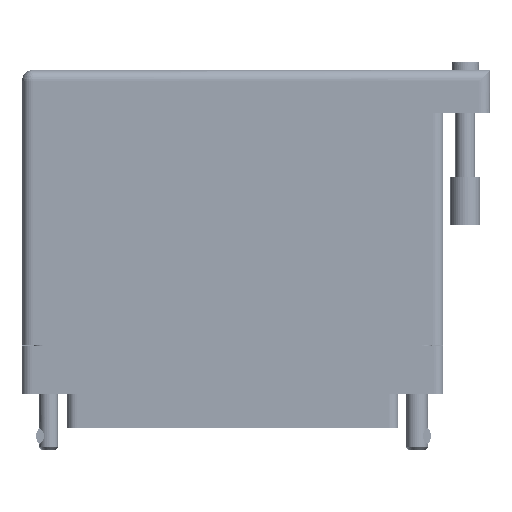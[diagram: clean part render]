
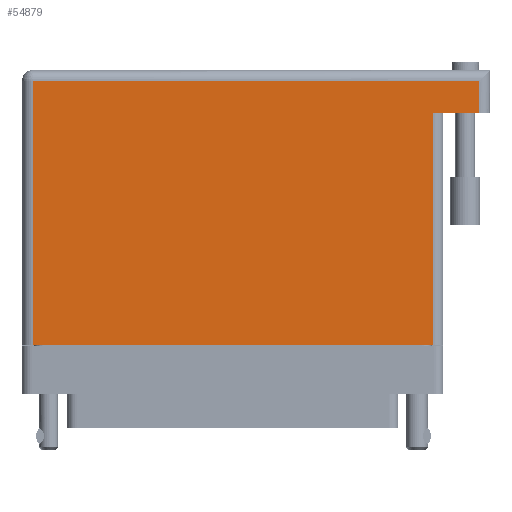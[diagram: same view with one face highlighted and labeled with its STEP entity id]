
A CAD part, front view. The second image highlights one B-rep face of the part: STEP entity #54879.
In plain terms, the highlighted face is planar.
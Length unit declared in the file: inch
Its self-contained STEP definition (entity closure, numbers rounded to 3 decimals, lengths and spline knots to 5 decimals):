
#2619 = DIRECTION ( 'NONE',  ( 0., 0., -1. ) ) ;
#3626 = CARTESIAN_POINT ( 'NONE',  ( 1.589, 1.605, 0.617 ) ) ;
#3721 = DIRECTION ( 'NONE',  ( 1., 0., 0. ) ) ;
#5409 = DIRECTION ( 'NONE',  ( -1., 0., 0. ) ) ;
#10530 = VECTOR ( 'NONE', #23652, 39.37008 ) ;
#10842 = LINE ( 'NONE', #23153, #66953 ) ;
#14920 = DIRECTION ( 'NONE',  ( -1., 0., 0. ) ) ;
#15500 = CARTESIAN_POINT ( 'NONE',  ( 1.289, -0.1, 0.617 ) ) ;
#17775 = CARTESIAN_POINT ( 'NONE',  ( 1.289, 1.395, 0.617 ) ) ;
#20350 = VERTEX_POINT ( 'NONE', #54851 ) ;
#20756 = EDGE_CURVE ( 'NONE', #31509, #25315, #49983, .T. ) ;
#21110 = LINE ( 'NONE', #66431, #63501 ) ;
#22135 = PLANE ( 'NONE',  #81626 ) ;
#23153 = CARTESIAN_POINT ( 'NONE',  ( 1.659, 1.395, 0.617 ) ) ;
#23652 = DIRECTION ( 'NONE',  ( 0., -1., 0. ) ) ;
#24788 = VERTEX_POINT ( 'NONE', #55376 ) ;
#25315 = VERTEX_POINT ( 'NONE', #38615 ) ;
#27882 = DIRECTION ( 'NONE',  ( 0., 1., 0. ) ) ;
#28761 = CARTESIAN_POINT ( 'NONE',  ( -1.289, 1.605, 0.617 ) ) ;
#31509 = VERTEX_POINT ( 'NONE', #15500 ) ;
#38293 = EDGE_LOOP ( 'NONE', ( #81218, #76548, #80251, #51467, #76571, #50069 ) ) ;
#38615 = CARTESIAN_POINT ( 'NONE',  ( 1.289, 1.395, 0.617 ) ) ;
#39125 = EDGE_CURVE ( 'NONE', #20350, #25315, #10842, .T. ) ;
#41628 = EDGE_CURVE ( 'NONE', #69132, #62494, #77031, .T. ) ;
#42671 = VECTOR ( 'NONE', #69472, 39.37008 ) ;
#49983 = LINE ( 'NONE', #17775, #42671 ) ;
#50069 = ORIENTED_EDGE ( 'NONE', *, *, #62685, .T. ) ;
#50326 = LINE ( 'NONE', #55845, #10530 ) ;
#50994 = VECTOR ( 'NONE', #5409, 39.37008 ) ;
#51467 = ORIENTED_EDGE ( 'NONE', *, *, #78425, .T. ) ;
#54851 = CARTESIAN_POINT ( 'NONE',  ( 1.589, 1.395, 0.617 ) ) ;
#54879 = ADVANCED_FACE ( 'NONE', ( #55159 ), #22135, .F. ) ;
#55159 = FACE_OUTER_BOUND ( 'NONE', #38293, .T. ) ;
#55376 = CARTESIAN_POINT ( 'NONE',  ( -1.289, -0.1, 0.617 ) ) ;
#55845 = CARTESIAN_POINT ( 'NONE',  ( -1.289, -0.1, 0.617 ) ) ;
#62494 = VERTEX_POINT ( 'NONE', #28761 ) ;
#62611 = EDGE_CURVE ( 'NONE', #24788, #31509, #74917, .T. ) ;
#62685 = EDGE_CURVE ( 'NONE', #62494, #24788, #50326, .T. ) ;
#63501 = VECTOR ( 'NONE', #27882, 39.37008 ) ;
#66431 = CARTESIAN_POINT ( 'NONE',  ( 1.589, 1.675, 0.617 ) ) ;
#66953 = VECTOR ( 'NONE', #68909, 39.37008 ) ;
#68909 = DIRECTION ( 'NONE',  ( -1., 0., 0. ) ) ;
#69132 = VERTEX_POINT ( 'NONE', #3626 ) ;
#69472 = DIRECTION ( 'NONE',  ( 0., 1., 0. ) ) ;
#72820 = VECTOR ( 'NONE', #3721, 39.37008 ) ;
#74917 = LINE ( 'NONE', #81711, #72820 ) ;
#76548 = ORIENTED_EDGE ( 'NONE', *, *, #20756, .T. ) ;
#76571 = ORIENTED_EDGE ( 'NONE', *, *, #41628, .T. ) ;
#76600 = CARTESIAN_POINT ( 'NONE',  ( -1.359, 1.605, 0.617 ) ) ;
#77031 = LINE ( 'NONE', #76600, #50994 ) ;
#78425 = EDGE_CURVE ( 'NONE', #20350, #69132, #21110, .T. ) ;
#80251 = ORIENTED_EDGE ( 'NONE', *, *, #39125, .F. ) ;
#81033 = CARTESIAN_POINT ( 'NONE',  ( -1.359, 1.675, 0.617 ) ) ;
#81218 = ORIENTED_EDGE ( 'NONE', *, *, #62611, .T. ) ;
#81626 = AXIS2_PLACEMENT_3D ( 'NONE', #81033, #2619, #14920 ) ;
#81711 = CARTESIAN_POINT ( 'NONE',  ( -1.359, -0.1, 0.617 ) ) ;
